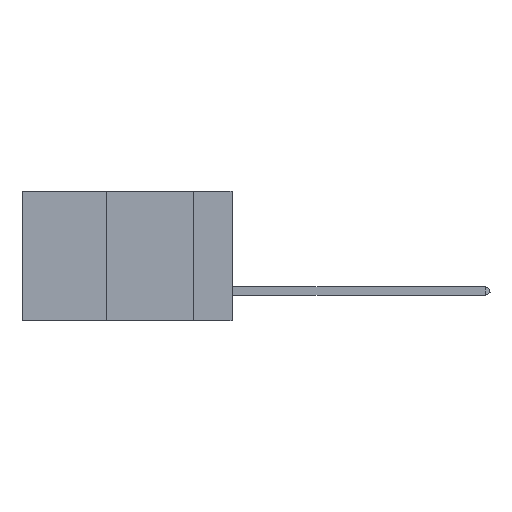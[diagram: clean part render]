
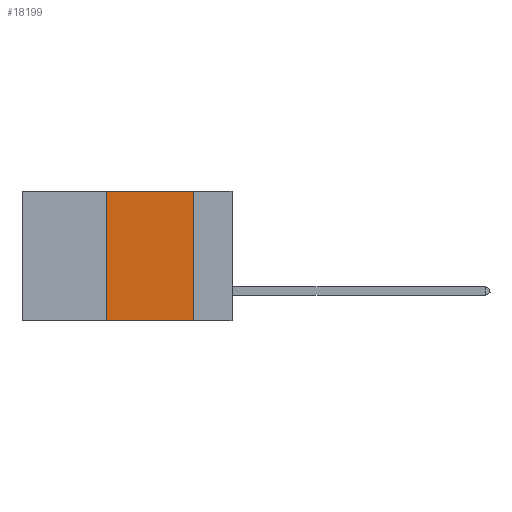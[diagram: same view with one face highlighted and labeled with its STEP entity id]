
A CAD part, left-side view. The second image highlights one B-rep face of the part: STEP entity #18199.
In plain terms, the highlighted planar face has unit normal (-1, 0, 0).
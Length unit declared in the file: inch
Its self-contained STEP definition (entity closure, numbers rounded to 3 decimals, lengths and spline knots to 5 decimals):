
#98 = VERTEX_POINT ( 'NONE', #13797 ) ;
#102 = EDGE_LOOP ( 'NONE', ( #19381, #19438, #27585, #8929 ) ) ;
#2042 = VECTOR ( 'NONE', #13871, 39.37008 ) ;
#8592 = CARTESIAN_POINT ( 'NONE',  ( 0., 0.6, -0.37 ) ) ;
#8929 = ORIENTED_EDGE ( 'NONE', *, *, #9490, .T. ) ;
#9490 = EDGE_CURVE ( 'NONE', #15890, #98, #12878, .T. ) ;
#9642 = EDGE_CURVE ( 'NONE', #15890, #10154, #16010, .T. ) ;
#10119 = DIRECTION ( 'NONE',  ( 0., -1., 0. ) ) ;
#10154 = VERTEX_POINT ( 'NONE', #27248 ) ;
#10270 = DIRECTION ( 'NONE',  ( 0., 0., -1. ) ) ;
#11199 = CARTESIAN_POINT ( 'NONE',  ( 0., 0.11, 0. ) ) ;
#12878 = LINE ( 'NONE', #8592, #2042 ) ;
#13797 = CARTESIAN_POINT ( 'NONE',  ( 0., 0.11, -0.37 ) ) ;
#13871 = DIRECTION ( 'NONE',  ( 0., -1., 0. ) ) ;
#14624 = EDGE_CURVE ( 'NONE', #10154, #19979, #35640, .T. ) ;
#15803 = PLANE ( 'NONE',  #32966 ) ;
#15890 = VERTEX_POINT ( 'NONE', #19115 ) ;
#16010 = LINE ( 'NONE', #18300, #19608 ) ;
#16046 = DIRECTION ( 'NONE',  ( 0., 0., 1. ) ) ;
#18199 = ADVANCED_FACE ( 'NONE', ( #22169 ), #15803, .F. ) ;
#18300 = CARTESIAN_POINT ( 'NONE',  ( 0., 0.36, 0. ) ) ;
#19011 = DIRECTION ( 'NONE',  ( 1., 0., 0. ) ) ;
#19115 = CARTESIAN_POINT ( 'NONE',  ( 0., 0.36, -0.37 ) ) ;
#19372 = VECTOR ( 'NONE', #21129, 39.37008 ) ;
#19381 = ORIENTED_EDGE ( 'NONE', *, *, #34857, .F. ) ;
#19438 = ORIENTED_EDGE ( 'NONE', *, *, #14624, .F. ) ;
#19608 = VECTOR ( 'NONE', #16046, 39.37008 ) ;
#19862 = LINE ( 'NONE', #32461, #19372 ) ;
#19979 = VERTEX_POINT ( 'NONE', #11199 ) ;
#21129 = DIRECTION ( 'NONE',  ( 0., 0., -1. ) ) ;
#22169 = FACE_OUTER_BOUND ( 'NONE', #102, .T. ) ;
#27042 = VECTOR ( 'NONE', #10119, 39.37008 ) ;
#27248 = CARTESIAN_POINT ( 'NONE',  ( 0., 0.36, 0. ) ) ;
#27446 = CARTESIAN_POINT ( 'NONE',  ( 0., 0.6, 0. ) ) ;
#27585 = ORIENTED_EDGE ( 'NONE', *, *, #9642, .F. ) ;
#32461 = CARTESIAN_POINT ( 'NONE',  ( 0., 0.11, 0. ) ) ;
#32966 = AXIS2_PLACEMENT_3D ( 'NONE', #27446, #19011, #10270 ) ;
#34857 = EDGE_CURVE ( 'NONE', #19979, #98, #19862, .T. ) ;
#35274 = CARTESIAN_POINT ( 'NONE',  ( 0., 0.6, 0. ) ) ;
#35640 = LINE ( 'NONE', #35274, #27042 ) ;
